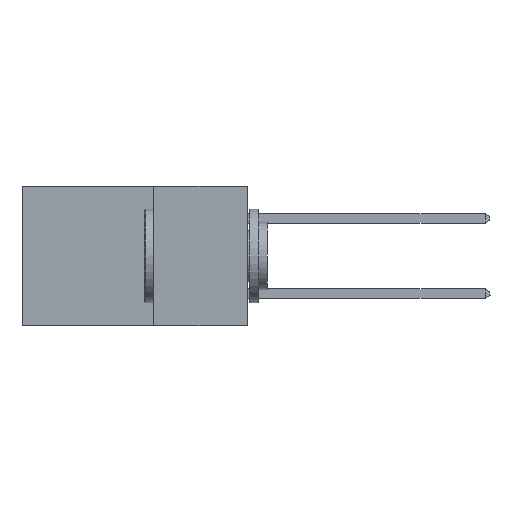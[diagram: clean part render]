
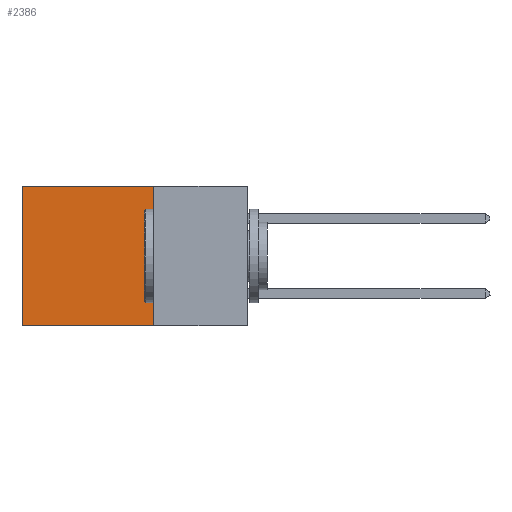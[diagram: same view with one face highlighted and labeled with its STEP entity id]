
A CAD part, left-side view. The second image highlights one B-rep face of the part: STEP entity #2386.
In plain terms, the highlighted planar face has unit normal (-1, 0, 0).
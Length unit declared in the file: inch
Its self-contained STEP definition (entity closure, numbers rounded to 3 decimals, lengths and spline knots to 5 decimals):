
#776 = VECTOR ( 'NONE', #7994, 39.37008 ) ;
#821 = VERTEX_POINT ( 'NONE', #11903 ) ;
#935 = FACE_OUTER_BOUND ( 'NONE', #5944, .T. ) ;
#1019 = CARTESIAN_POINT ( 'NONE',  ( 0.298, 0.25, 0. ) ) ;
#1097 = LINE ( 'NONE', #5832, #5285 ) ;
#1501 = EDGE_CURVE ( 'NONE', #7869, #821, #7172, .T. ) ;
#1528 = CARTESIAN_POINT ( 'NONE',  ( 0.298, 0.6, 0. ) ) ;
#1757 = EDGE_CURVE ( 'NONE', #7869, #3912, #1097, .T. ) ;
#1908 = VERTEX_POINT ( 'NONE', #8143 ) ;
#2097 = DIRECTION ( 'NONE',  ( 1., 0., 0. ) ) ;
#2140 = CARTESIAN_POINT ( 'NONE',  ( 0.298, 0.25, 0. ) ) ;
#2386 = ADVANCED_FACE ( 'NONE', ( #935 ), #7634, .F. ) ;
#2906 = ORIENTED_EDGE ( 'NONE', *, *, #8137, .T. ) ;
#3479 = VECTOR ( 'NONE', #10879, 39.37008 ) ;
#3780 = LINE ( 'NONE', #11748, #3479 ) ;
#3912 = VERTEX_POINT ( 'NONE', #4542 ) ;
#3976 = CARTESIAN_POINT ( 'NONE',  ( 0.298, 0.25, 0. ) ) ;
#4013 = EDGE_CURVE ( 'NONE', #3912, #1908, #3780, .T. ) ;
#4166 = ORIENTED_EDGE ( 'NONE', *, *, #1501, .T. ) ;
#4542 = CARTESIAN_POINT ( 'NONE',  ( 0.298, 0.25, -0.37 ) ) ;
#5285 = VECTOR ( 'NONE', #7645, 39.37008 ) ;
#5832 = CARTESIAN_POINT ( 'NONE',  ( 0.298, 0.25, 0. ) ) ;
#5944 = EDGE_LOOP ( 'NONE', ( #2906, #9333, #10328, #4166 ) ) ;
#7172 = LINE ( 'NONE', #1019, #10800 ) ;
#7422 = AXIS2_PLACEMENT_3D ( 'NONE', #2140, #2097, #10311 ) ;
#7634 = PLANE ( 'NONE',  #7422 ) ;
#7645 = DIRECTION ( 'NONE',  ( 0., 0., -1. ) ) ;
#7869 = VERTEX_POINT ( 'NONE', #3976 ) ;
#7994 = DIRECTION ( 'NONE',  ( 0., 0., -1. ) ) ;
#8137 = EDGE_CURVE ( 'NONE', #821, #1908, #10612, .T. ) ;
#8143 = CARTESIAN_POINT ( 'NONE',  ( 0.298, 0.6, -0.37 ) ) ;
#9333 = ORIENTED_EDGE ( 'NONE', *, *, #4013, .F. ) ;
#9400 = DIRECTION ( 'NONE',  ( 0., 1., 0. ) ) ;
#10311 = DIRECTION ( 'NONE',  ( 0., 0., -1. ) ) ;
#10328 = ORIENTED_EDGE ( 'NONE', *, *, #1757, .F. ) ;
#10612 = LINE ( 'NONE', #1528, #776 ) ;
#10800 = VECTOR ( 'NONE', #9400, 39.37008 ) ;
#10879 = DIRECTION ( 'NONE',  ( 0., 1., 0. ) ) ;
#11748 = CARTESIAN_POINT ( 'NONE',  ( 0.298, 0.25, -0.37 ) ) ;
#11903 = CARTESIAN_POINT ( 'NONE',  ( 0.298, 0.6, 0. ) ) ;
